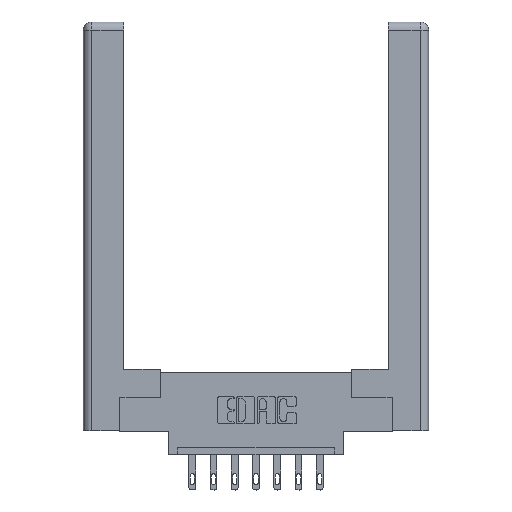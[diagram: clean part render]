
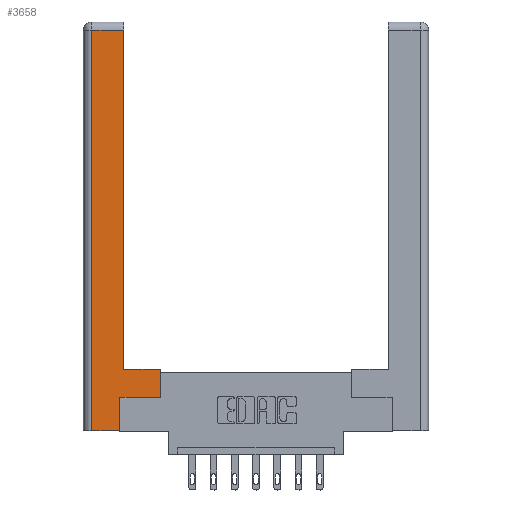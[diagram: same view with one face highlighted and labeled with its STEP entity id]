
A CAD part, top view. The second image highlights one B-rep face of the part: STEP entity #3658.
In plain terms, the highlighted planar face has unit normal (0, 0, 1).
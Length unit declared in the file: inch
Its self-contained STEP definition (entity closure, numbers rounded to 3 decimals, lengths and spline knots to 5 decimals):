
#206 = CARTESIAN_POINT ( 'NONE',  ( 0.295, 2.94, 0. ) ) ;
#344 = ORIENTED_EDGE ( 'NONE', *, *, #8693, .T. ) ;
#760 = AXIS2_PLACEMENT_3D ( 'NONE', #4714, #7758, #11598 ) ;
#885 = EDGE_CURVE ( 'NONE', #2982, #12077, #5995, .T. ) ;
#1130 = EDGE_CURVE ( 'NONE', #2367, #11232, #9123, .T. ) ;
#1443 = ORIENTED_EDGE ( 'NONE', *, *, #5697, .T. ) ;
#1465 = CARTESIAN_POINT ( 'NONE',  ( 0.0615, 2.94, 0. ) ) ;
#2367 = VERTEX_POINT ( 'NONE', #1465 ) ;
#2445 = CARTESIAN_POINT ( 'NONE',  ( 0.265, 0., 0. ) ) ;
#2889 = FACE_OUTER_BOUND ( 'NONE', #4857, .T. ) ;
#2972 = DIRECTION ( 'NONE',  ( 1., 0., 0. ) ) ;
#2982 = VERTEX_POINT ( 'NONE', #7331 ) ;
#3048 = DIRECTION ( 'NONE',  ( 0., 1., 0. ) ) ;
#3202 = LINE ( 'NONE', #9543, #3510 ) ;
#3313 = CARTESIAN_POINT ( 'NONE',  ( 0.565, 0.45, 0. ) ) ;
#3327 = VECTOR ( 'NONE', #8079, 39.37008 ) ;
#3464 = CARTESIAN_POINT ( 'NONE',  ( 0.0615, 2.94, 0. ) ) ;
#3510 = VECTOR ( 'NONE', #2972, 39.37008 ) ;
#3630 = ORIENTED_EDGE ( 'NONE', *, *, #8394, .T. ) ;
#3658 = ADVANCED_FACE ( 'NONE', ( #2889 ), #8669, .F. ) ;
#3699 = EDGE_CURVE ( 'NONE', #4460, #2982, #3202, .T. ) ;
#3848 = VECTOR ( 'NONE', #6428, 39.37008 ) ;
#4010 = VECTOR ( 'NONE', #5518, 39.37008 ) ;
#4224 = ORIENTED_EDGE ( 'NONE', *, *, #1130, .T. ) ;
#4234 = LINE ( 'NONE', #5343, #3327 ) ;
#4421 = VERTEX_POINT ( 'NONE', #5584 ) ;
#4460 = VERTEX_POINT ( 'NONE', #7610 ) ;
#4625 = VECTOR ( 'NONE', #3048, 39.37008 ) ;
#4714 = CARTESIAN_POINT ( 'NONE',  ( 0., 0., 0. ) ) ;
#4775 = EDGE_CURVE ( 'NONE', #12077, #4421, #4234, .T. ) ;
#4857 = EDGE_LOOP ( 'NONE', ( #344, #3630, #4224, #1443, #9624, #5775, #7377, #5432 ) ) ;
#4963 = LINE ( 'NONE', #9007, #8740 ) ;
#5011 = CARTESIAN_POINT ( 'NONE',  ( 0.0615, 0., 0. ) ) ;
#5343 = CARTESIAN_POINT ( 'NONE',  ( 0.295, 0.45, 0. ) ) ;
#5432 = ORIENTED_EDGE ( 'NONE', *, *, #4775, .T. ) ;
#5518 = DIRECTION ( 'NONE',  ( 0., -1., 0. ) ) ;
#5584 = CARTESIAN_POINT ( 'NONE',  ( 0.295, 0.45, 0. ) ) ;
#5697 = EDGE_CURVE ( 'NONE', #11232, #11282, #5885, .T. ) ;
#5775 = ORIENTED_EDGE ( 'NONE', *, *, #3699, .T. ) ;
#5792 = EDGE_CURVE ( 'NONE', #11282, #4460, #4963, .T. ) ;
#5885 = LINE ( 'NONE', #10947, #7101 ) ;
#5968 = VECTOR ( 'NONE', #6921, 39.37008 ) ;
#5995 = LINE ( 'NONE', #6874, #4625 ) ;
#6428 = DIRECTION ( 'NONE',  ( -1., 0., 0. ) ) ;
#6791 = VERTEX_POINT ( 'NONE', #206 ) ;
#6874 = CARTESIAN_POINT ( 'NONE',  ( 0.565, 0.45, 0. ) ) ;
#6921 = DIRECTION ( 'NONE',  ( 0., 1., 0. ) ) ;
#7101 = VECTOR ( 'NONE', #8021, 39.37008 ) ;
#7331 = CARTESIAN_POINT ( 'NONE',  ( 0.565, 0.245, 0. ) ) ;
#7377 = ORIENTED_EDGE ( 'NONE', *, *, #885, .T. ) ;
#7610 = CARTESIAN_POINT ( 'NONE',  ( 0.265, 0.245, 0. ) ) ;
#7758 = DIRECTION ( 'NONE',  ( 0., 0., -1. ) ) ;
#8021 = DIRECTION ( 'NONE',  ( 1., 0., 0. ) ) ;
#8079 = DIRECTION ( 'NONE',  ( -1., 0., 0. ) ) ;
#8394 = EDGE_CURVE ( 'NONE', #6791, #2367, #9701, .T. ) ;
#8512 = LINE ( 'NONE', #8864, #5968 ) ;
#8669 = PLANE ( 'NONE',  #760 ) ;
#8693 = EDGE_CURVE ( 'NONE', #4421, #6791, #8512, .T. ) ;
#8740 = VECTOR ( 'NONE', #9976, 39.37008 ) ;
#8864 = CARTESIAN_POINT ( 'NONE',  ( 0.295, 3., 0. ) ) ;
#9007 = CARTESIAN_POINT ( 'NONE',  ( 0.265, 0.245, 0. ) ) ;
#9123 = LINE ( 'NONE', #10292, #4010 ) ;
#9543 = CARTESIAN_POINT ( 'NONE',  ( 0.565, 0.245, 0. ) ) ;
#9624 = ORIENTED_EDGE ( 'NONE', *, *, #5792, .T. ) ;
#9701 = LINE ( 'NONE', #3464, #3848 ) ;
#9976 = DIRECTION ( 'NONE',  ( 0., 1., 0. ) ) ;
#10292 = CARTESIAN_POINT ( 'NONE',  ( 0.0615, 0., 0. ) ) ;
#10947 = CARTESIAN_POINT ( 'NONE',  ( 0.265, 0., 0. ) ) ;
#11232 = VERTEX_POINT ( 'NONE', #5011 ) ;
#11282 = VERTEX_POINT ( 'NONE', #2445 ) ;
#11598 = DIRECTION ( 'NONE',  ( -1., 0., 0. ) ) ;
#12077 = VERTEX_POINT ( 'NONE', #3313 ) ;
